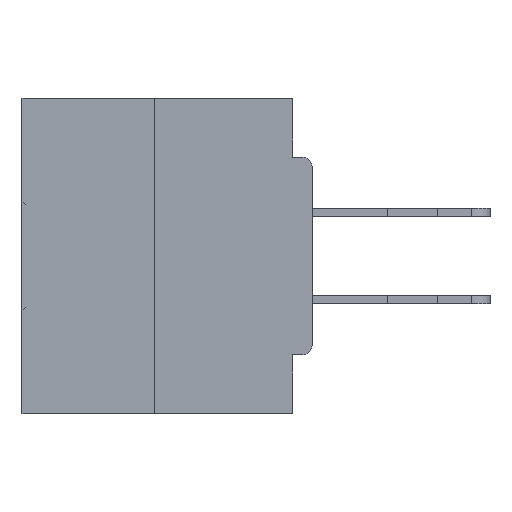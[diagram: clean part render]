
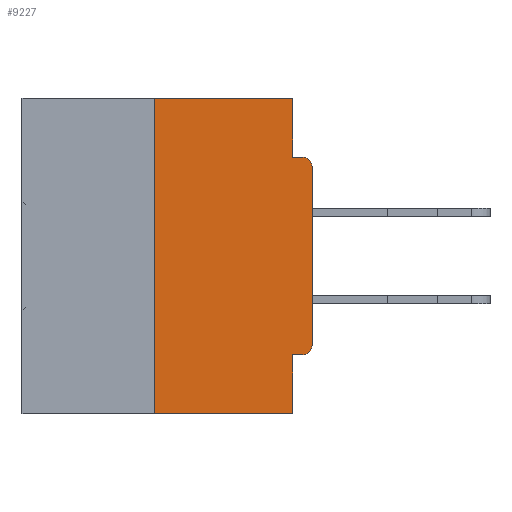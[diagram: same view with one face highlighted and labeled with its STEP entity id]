
A CAD part, left-side view. The second image highlights one B-rep face of the part: STEP entity #9227.
In plain terms, the highlighted planar face has unit normal (-1, 0, 0).
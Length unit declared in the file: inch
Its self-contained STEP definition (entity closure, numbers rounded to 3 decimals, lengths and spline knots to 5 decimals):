
#56 = CARTESIAN_POINT ( 'NONE',  ( 0., 0.015, -0.0935 ) ) ;
#667 = LINE ( 'NONE', #25234, #36417 ) ;
#1328 = VECTOR ( 'NONE', #18896, 39.37008 ) ;
#2302 = VERTEX_POINT ( 'NONE', #37790 ) ;
#3530 = VERTEX_POINT ( 'NONE', #25002 ) ;
#4692 = EDGE_CURVE ( 'NONE', #9838, #3530, #42814, .T. ) ;
#5230 = ORIENTED_EDGE ( 'NONE', *, *, #6394, .T. ) ;
#5374 = ORIENTED_EDGE ( 'NONE', *, *, #34811, .F. ) ;
#6394 = EDGE_CURVE ( 'NONE', #31278, #18388, #39996, .T. ) ;
#6574 = ORIENTED_EDGE ( 'NONE', *, *, #28815, .T. ) ;
#8624 = ORIENTED_EDGE ( 'NONE', *, *, #19638, .F. ) ;
#8981 = DIRECTION ( 'NONE',  ( 0., 0., -1. ) ) ;
#9014 = CARTESIAN_POINT ( 'NONE',  ( 0., 0.46, 0. ) ) ;
#9227 = ADVANCED_FACE ( 'NONE', ( #22510 ), #37810, .F. ) ;
#9294 = VECTOR ( 'NONE', #30382, 39.37008 ) ;
#9838 = VERTEX_POINT ( 'NONE', #16805 ) ;
#10172 = EDGE_CURVE ( 'NONE', #36651, #2302, #27303, .T. ) ;
#10599 = ORIENTED_EDGE ( 'NONE', *, *, #11152, .T. ) ;
#11152 = EDGE_CURVE ( 'NONE', #2302, #26431, #21481, .T. ) ;
#11868 = DIRECTION ( 'NONE',  ( 0., 0., -1. ) ) ;
#13174 = DIRECTION ( 'NONE',  ( 0., 0., -1. ) ) ;
#13797 = LINE ( 'NONE', #29078, #1328 ) ;
#13927 = CARTESIAN_POINT ( 'NONE',  ( 0., 0.46, 0. ) ) ;
#14241 = CARTESIAN_POINT ( 'NONE',  ( 0., 0.25, 0. ) ) ;
#14332 = CARTESIAN_POINT ( 'NONE',  ( 0., 0.031, -0.4065 ) ) ;
#14701 = DIRECTION ( 'NONE',  ( 0., 0., 1. ) ) ;
#15224 = VECTOR ( 'NONE', #15657, 39.37008 ) ;
#15657 = DIRECTION ( 'NONE',  ( 0., -1., 0. ) ) ;
#16433 = AXIS2_PLACEMENT_3D ( 'NONE', #42362, #29029, #11868 ) ;
#16602 = VERTEX_POINT ( 'NONE', #42358 ) ;
#16729 = DIRECTION ( 'NONE',  ( 0., -1., 0. ) ) ;
#16805 = CARTESIAN_POINT ( 'NONE',  ( 0., 0.25, 0. ) ) ;
#18011 = VERTEX_POINT ( 'NONE', #22395 ) ;
#18388 = VERTEX_POINT ( 'NONE', #38973 ) ;
#18811 = CARTESIAN_POINT ( 'NONE',  ( 0., 0.25, -0.5 ) ) ;
#18896 = DIRECTION ( 'NONE',  ( 0., 1., 0. ) ) ;
#19638 = EDGE_CURVE ( 'NONE', #16602, #26431, #25745, .T. ) ;
#19963 = CARTESIAN_POINT ( 'NONE',  ( 0., 0.031, 0. ) ) ;
#20403 = LINE ( 'NONE', #19963, #23154 ) ;
#20906 = DIRECTION ( 'NONE',  ( 0., 0., -1. ) ) ;
#21481 = CIRCLE ( 'NONE', #16433, 0.015 ) ;
#21965 = VECTOR ( 'NONE', #16729, 39.37008 ) ;
#22395 = CARTESIAN_POINT ( 'NONE',  ( 0., 0.015, -0.4065 ) ) ;
#22510 = FACE_OUTER_BOUND ( 'NONE', #34064, .T. ) ;
#23154 = VECTOR ( 'NONE', #13174, 39.37008 ) ;
#23487 = EDGE_CURVE ( 'NONE', #3530, #16602, #20403, .T. ) ;
#25002 = CARTESIAN_POINT ( 'NONE',  ( 0., 0.031, 0. ) ) ;
#25234 = CARTESIAN_POINT ( 'NONE',  ( 0., 0.031, -0.5 ) ) ;
#25745 = LINE ( 'NONE', #27035, #21965 ) ;
#26431 = VERTEX_POINT ( 'NONE', #56 ) ;
#26445 = VERTEX_POINT ( 'NONE', #14332 ) ;
#27035 = CARTESIAN_POINT ( 'NONE',  ( 0., 0., -0.0935 ) ) ;
#27303 = LINE ( 'NONE', #44426, #35422 ) ;
#27318 = DIRECTION ( 'NONE',  ( 0., 0., 1. ) ) ;
#27533 = ORIENTED_EDGE ( 'NONE', *, *, #4692, .F. ) ;
#28815 = EDGE_CURVE ( 'NONE', #18011, #36651, #29283, .T. ) ;
#29029 = DIRECTION ( 'NONE',  ( -1., 0., 0. ) ) ;
#29078 = CARTESIAN_POINT ( 'NONE',  ( 0., 0., -0.4065 ) ) ;
#29283 = CIRCLE ( 'NONE', #40001, 0.015 ) ;
#30382 = DIRECTION ( 'NONE',  ( 0., -1., 0. ) ) ;
#31278 = VERTEX_POINT ( 'NONE', #18811 ) ;
#31813 = CARTESIAN_POINT ( 'NONE',  ( 0., 0.46, -0.5 ) ) ;
#32556 = ORIENTED_EDGE ( 'NONE', *, *, #32679, .F. ) ;
#32679 = EDGE_CURVE ( 'NONE', #18011, #26445, #13797, .T. ) ;
#32931 = CARTESIAN_POINT ( 'NONE',  ( 0., 0.015, -0.3915 ) ) ;
#33641 = ORIENTED_EDGE ( 'NONE', *, *, #42287, .F. ) ;
#34064 = EDGE_LOOP ( 'NONE', ( #27533, #5374, #5230, #33641, #32556, #6574, #41500, #10599, #8624, #42952 ) ) ;
#34811 = EDGE_CURVE ( 'NONE', #31278, #9838, #36846, .T. ) ;
#35422 = VECTOR ( 'NONE', #27318, 39.37008 ) ;
#36417 = VECTOR ( 'NONE', #8981, 39.37008 ) ;
#36651 = VERTEX_POINT ( 'NONE', #41601 ) ;
#36846 = LINE ( 'NONE', #14241, #42734 ) ;
#37314 = AXIS2_PLACEMENT_3D ( 'NONE', #13927, #38417, #20906 ) ;
#37790 = CARTESIAN_POINT ( 'NONE',  ( 0., 0., -0.1085 ) ) ;
#37810 = PLANE ( 'NONE',  #37314 ) ;
#38417 = DIRECTION ( 'NONE',  ( 1., 0., 0. ) ) ;
#38973 = CARTESIAN_POINT ( 'NONE',  ( 0., 0.031, -0.5 ) ) ;
#39996 = LINE ( 'NONE', #31813, #15224 ) ;
#40001 = AXIS2_PLACEMENT_3D ( 'NONE', #32931, #40067, #43384 ) ;
#40067 = DIRECTION ( 'NONE',  ( -1., 0., 0. ) ) ;
#41500 = ORIENTED_EDGE ( 'NONE', *, *, #10172, .T. ) ;
#41601 = CARTESIAN_POINT ( 'NONE',  ( 0., 0., -0.3915 ) ) ;
#42287 = EDGE_CURVE ( 'NONE', #26445, #18388, #667, .T. ) ;
#42358 = CARTESIAN_POINT ( 'NONE',  ( 0., 0.031, -0.0935 ) ) ;
#42362 = CARTESIAN_POINT ( 'NONE',  ( 0., 0.015, -0.1085 ) ) ;
#42734 = VECTOR ( 'NONE', #14701, 39.37008 ) ;
#42814 = LINE ( 'NONE', #9014, #9294 ) ;
#42952 = ORIENTED_EDGE ( 'NONE', *, *, #23487, .F. ) ;
#43384 = DIRECTION ( 'NONE',  ( 0., 0., -1. ) ) ;
#44426 = CARTESIAN_POINT ( 'NONE',  ( 0., 0., 0. ) ) ;
